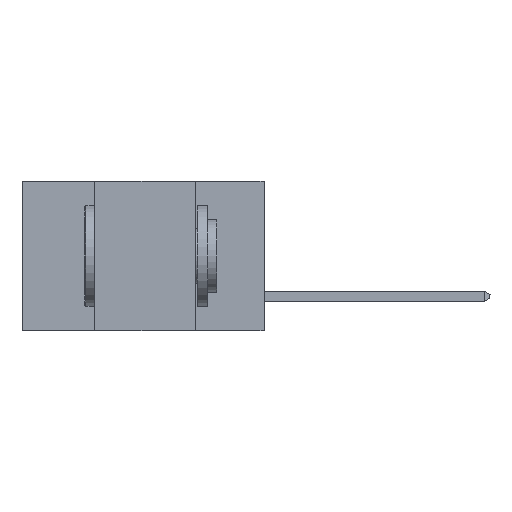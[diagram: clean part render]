
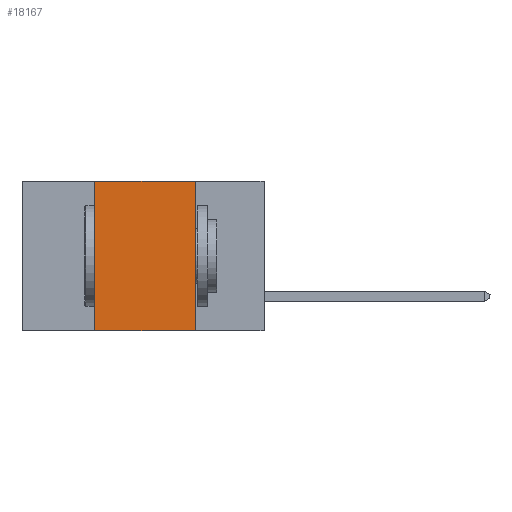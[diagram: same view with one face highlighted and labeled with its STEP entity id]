
A CAD part, left-side view. The second image highlights one B-rep face of the part: STEP entity #18167.
In plain terms, the highlighted planar face has unit normal (-1, 0, 0).
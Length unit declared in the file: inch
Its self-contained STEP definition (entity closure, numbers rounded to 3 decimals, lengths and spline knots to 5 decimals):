
#813 = DIRECTION ( 'NONE',  ( 1., 0., 0. ) ) ;
#1713 = LINE ( 'NONE', #18138, #4119 ) ;
#1816 = VERTEX_POINT ( 'NONE', #9974 ) ;
#1896 = DIRECTION ( 'NONE',  ( 0., -1., 0. ) ) ;
#2040 = EDGE_CURVE ( 'NONE', #17916, #27752, #9563, .T. ) ;
#2396 = ORIENTED_EDGE ( 'NONE', *, *, #22188, .F. ) ;
#2914 = CARTESIAN_POINT ( 'NONE',  ( 0., 0.6, -0.37 ) ) ;
#3104 = DIRECTION ( 'NONE',  ( 0., -1., 0. ) ) ;
#4119 = VECTOR ( 'NONE', #26932, 39.37008 ) ;
#4266 = CARTESIAN_POINT ( 'NONE',  ( 0., 0.42, -0.37 ) ) ;
#5463 = CARTESIAN_POINT ( 'NONE',  ( 0., 0.17, -0.37 ) ) ;
#7345 = CARTESIAN_POINT ( 'NONE',  ( 0., 0.6, 0. ) ) ;
#7421 = FACE_OUTER_BOUND ( 'NONE', #25860, .T. ) ;
#8365 = DIRECTION ( 'NONE',  ( 0., 0., 1. ) ) ;
#9563 = LINE ( 'NONE', #2914, #22940 ) ;
#9974 = CARTESIAN_POINT ( 'NONE',  ( 0., 0.42, 0. ) ) ;
#10666 = ORIENTED_EDGE ( 'NONE', *, *, #13324, .F. ) ;
#11531 = AXIS2_PLACEMENT_3D ( 'NONE', #7345, #813, #22838 ) ;
#12367 = CARTESIAN_POINT ( 'NONE',  ( 0., 0.17, 0. ) ) ;
#12992 = ORIENTED_EDGE ( 'NONE', *, *, #2040, .T. ) ;
#13324 = EDGE_CURVE ( 'NONE', #1816, #16047, #27574, .T. ) ;
#14424 = ORIENTED_EDGE ( 'NONE', *, *, #16809, .F. ) ;
#16047 = VERTEX_POINT ( 'NONE', #12367 ) ;
#16303 = PLANE ( 'NONE',  #11531 ) ;
#16809 = EDGE_CURVE ( 'NONE', #16047, #27752, #1713, .T. ) ;
#17916 = VERTEX_POINT ( 'NONE', #4266 ) ;
#18138 = CARTESIAN_POINT ( 'NONE',  ( 0., 0.17, 0. ) ) ;
#18167 = ADVANCED_FACE ( 'NONE', ( #7421 ), #16303, .F. ) ;
#21189 = VECTOR ( 'NONE', #8365, 39.37008 ) ;
#22188 = EDGE_CURVE ( 'NONE', #17916, #1816, #24644, .T. ) ;
#22838 = DIRECTION ( 'NONE',  ( 0., 0., -1. ) ) ;
#22940 = VECTOR ( 'NONE', #3104, 39.37008 ) ;
#23567 = CARTESIAN_POINT ( 'NONE',  ( 0., 0.42, 0. ) ) ;
#24644 = LINE ( 'NONE', #23567, #21189 ) ;
#25493 = VECTOR ( 'NONE', #1896, 39.37008 ) ;
#25720 = CARTESIAN_POINT ( 'NONE',  ( 0., 0.6, 0. ) ) ;
#25860 = EDGE_LOOP ( 'NONE', ( #14424, #10666, #2396, #12992 ) ) ;
#26932 = DIRECTION ( 'NONE',  ( 0., 0., -1. ) ) ;
#27574 = LINE ( 'NONE', #25720, #25493 ) ;
#27752 = VERTEX_POINT ( 'NONE', #5463 ) ;
